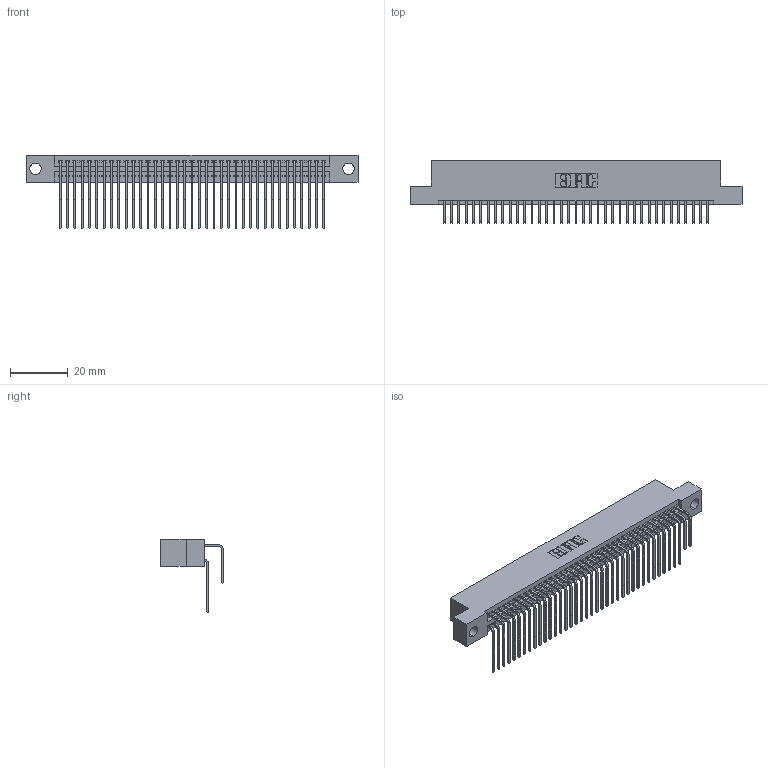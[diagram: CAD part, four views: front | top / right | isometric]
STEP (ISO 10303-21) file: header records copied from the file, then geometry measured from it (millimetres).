
FILE_DESCRIPTION (( 'STEP AP203' ), '1' );
FILE_NAME ('395-074-558-204.STEP', '2021-06-17T05:42:43', ( '' ), ( '' ), 'SwSTEP 2.0', 'SolidWorks 2020', '' );
FILE_SCHEMA (( 'CONFIG_CONTROL_DESIGN' ));
Length unit declared in the file: inch
Products named in the file (4): 345 Part_Flush Mounting Lugs - 0.156 Dia-TI; 345-292-001_558 Tail - 2; 345-292-001_558 559 Tail - 1; 395-074-558-204
Assembly tree (75 placements, depth 2):
  395-074-558-204
    345 Part_Flush Mounting Lugs - 0.156 Dia-TI
    345-292-001_558 559 Tail - 1  x37
    345-292-001_558 Tail - 2  x37
Bounding box: 115.19 x 21.83 x 25.53 mm (x, y, z)
Volume: 11464.1 mm3; surface area: 18708 mm2
Topology: 75 solids, 75 shells, 3988 faces, 11847 edges, 7798 vertices
Faces by surface type: plane 2684, cylinder 1304
Entity records: 31775 total; most frequent: CARTESIAN_POINT 5381, ORIENTED_EDGE 5262, DIRECTION 4723, EDGE_CURVE 2631, VECTOR 2311, LINE 2311, VERTEX_POINT 1750, AXIS2_PLACEMENT_3D 1206
